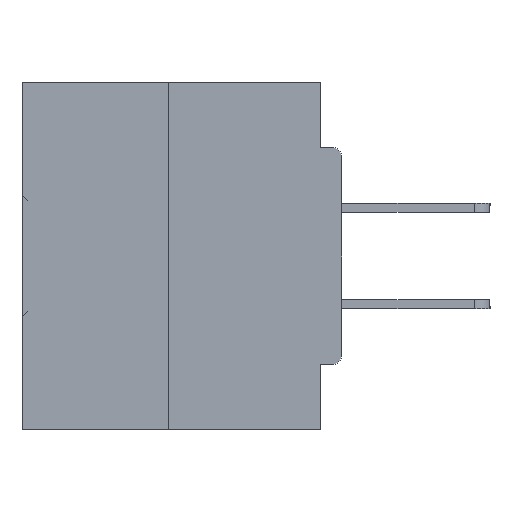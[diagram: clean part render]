
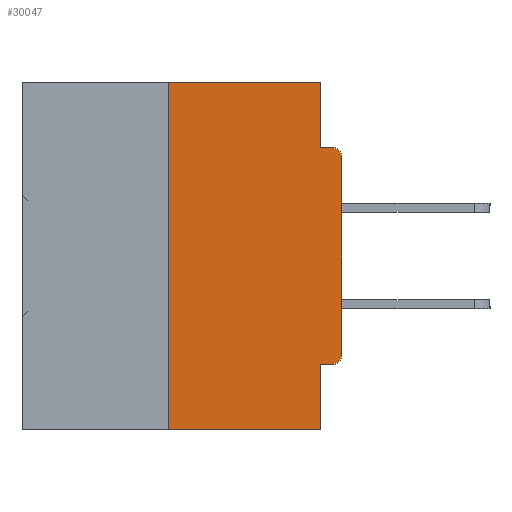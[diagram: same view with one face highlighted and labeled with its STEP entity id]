
A CAD part, left-side view. The second image highlights one B-rep face of the part: STEP entity #30047.
In plain terms, the highlighted planar face has unit normal (-1, 0, 0).
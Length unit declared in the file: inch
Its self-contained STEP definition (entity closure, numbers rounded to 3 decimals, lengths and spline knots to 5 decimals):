
#75 = ORIENTED_EDGE ( 'NONE', *, *, #35753, .F. ) ;
#793 = CARTESIAN_POINT ( 'NONE',  ( 0., 0.031, -0.0935 ) ) ;
#1240 = DIRECTION ( 'NONE',  ( 0., 0., 1. ) ) ;
#2278 = LINE ( 'NONE', #16675, #15530 ) ;
#2616 = VECTOR ( 'NONE', #43213, 39.37008 ) ;
#3412 = EDGE_CURVE ( 'NONE', #6064, #9976, #33629, .T. ) ;
#3781 = VECTOR ( 'NONE', #18982, 39.37008 ) ;
#4092 = CARTESIAN_POINT ( 'NONE',  ( 0., 0.25, 0. ) ) ;
#4139 = DIRECTION ( 'NONE',  ( 0., -1., 0. ) ) ;
#4508 = VERTEX_POINT ( 'NONE', #6081 ) ;
#4993 = CARTESIAN_POINT ( 'NONE',  ( 0., 0.25, 0. ) ) ;
#5034 = CARTESIAN_POINT ( 'NONE',  ( 0., 0., -0.3915 ) ) ;
#5086 = DIRECTION ( 'NONE',  ( 0., 1., 0. ) ) ;
#5139 = FACE_OUTER_BOUND ( 'NONE', #24367, .T. ) ;
#5368 = DIRECTION ( 'NONE',  ( 0., 0., -1. ) ) ;
#6064 = VERTEX_POINT ( 'NONE', #5034 ) ;
#6081 = CARTESIAN_POINT ( 'NONE',  ( 0., 0.25, -0.5 ) ) ;
#7770 = EDGE_CURVE ( 'NONE', #8188, #32114, #13104, .T. ) ;
#7917 = LINE ( 'NONE', #37010, #18830 ) ;
#8063 = VERTEX_POINT ( 'NONE', #11401 ) ;
#8188 = VERTEX_POINT ( 'NONE', #22750 ) ;
#8562 = ORIENTED_EDGE ( 'NONE', *, *, #7770, .F. ) ;
#8896 = CIRCLE ( 'NONE', #14152, 0.015 ) ;
#9626 = DIRECTION ( 'NONE',  ( 1., 0., 0. ) ) ;
#9976 = VERTEX_POINT ( 'NONE', #10866 ) ;
#10424 = DIRECTION ( 'NONE',  ( -1., 0., 0. ) ) ;
#10453 = CARTESIAN_POINT ( 'NONE',  ( 0., 0.015, -0.3915 ) ) ;
#10866 = CARTESIAN_POINT ( 'NONE',  ( 0., 0., -0.1085 ) ) ;
#11401 = CARTESIAN_POINT ( 'NONE',  ( 0., 0.031, -0.5 ) ) ;
#12155 = VECTOR ( 'NONE', #5086, 39.37008 ) ;
#12430 = ORIENTED_EDGE ( 'NONE', *, *, #3412, .T. ) ;
#13104 = LINE ( 'NONE', #37975, #12155 ) ;
#13108 = EDGE_CURVE ( 'NONE', #21368, #27125, #28758, .T. ) ;
#13872 = CIRCLE ( 'NONE', #43394, 0.015 ) ;
#14152 = AXIS2_PLACEMENT_3D ( 'NONE', #24622, #10424, #43067 ) ;
#14954 = EDGE_CURVE ( 'NONE', #4508, #8063, #7917, .T. ) ;
#14983 = CARTESIAN_POINT ( 'NONE',  ( 0., 0.031, 0. ) ) ;
#15158 = DIRECTION ( 'NONE',  ( 0., 0., -1. ) ) ;
#15449 = EDGE_CURVE ( 'NONE', #27125, #32962, #36286, .T. ) ;
#15530 = VECTOR ( 'NONE', #15158, 39.37008 ) ;
#15756 = CARTESIAN_POINT ( 'NONE',  ( 0., 0.46, 0. ) ) ;
#15834 = DIRECTION ( 'NONE',  ( 0., 0., 1. ) ) ;
#16675 = CARTESIAN_POINT ( 'NONE',  ( 0., 0.031, -0.5 ) ) ;
#16897 = VECTOR ( 'NONE', #15834, 39.37008 ) ;
#18085 = VERTEX_POINT ( 'NONE', #39453 ) ;
#18830 = VECTOR ( 'NONE', #4139, 39.37008 ) ;
#18982 = DIRECTION ( 'NONE',  ( 0., 0., -1. ) ) ;
#20899 = ORIENTED_EDGE ( 'NONE', *, *, #44696, .F. ) ;
#21368 = VERTEX_POINT ( 'NONE', #4092 ) ;
#21892 = CARTESIAN_POINT ( 'NONE',  ( 0., 0.46, 0. ) ) ;
#21926 = ORIENTED_EDGE ( 'NONE', *, *, #15449, .F. ) ;
#22748 = CARTESIAN_POINT ( 'NONE',  ( 0., 0., 0. ) ) ;
#22750 = CARTESIAN_POINT ( 'NONE',  ( 0., 0.015, -0.4065 ) ) ;
#23289 = CARTESIAN_POINT ( 'NONE',  ( 0., 0.031, 0. ) ) ;
#24070 = CARTESIAN_POINT ( 'NONE',  ( 0., 0., -0.0935 ) ) ;
#24367 = EDGE_LOOP ( 'NONE', ( #28938, #75, #28077, #20899, #8562, #33001, #12430, #25408, #25571, #21926 ) ) ;
#24622 = CARTESIAN_POINT ( 'NONE',  ( 0., 0.015, -0.1085 ) ) ;
#24874 = DIRECTION ( 'NONE',  ( -1., 0., 0. ) ) ;
#25199 = VECTOR ( 'NONE', #38513, 39.37008 ) ;
#25408 = ORIENTED_EDGE ( 'NONE', *, *, #38460, .T. ) ;
#25571 = ORIENTED_EDGE ( 'NONE', *, *, #40719, .F. ) ;
#27125 = VERTEX_POINT ( 'NONE', #23289 ) ;
#28077 = ORIENTED_EDGE ( 'NONE', *, *, #14954, .T. ) ;
#28758 = LINE ( 'NONE', #21892, #2616 ) ;
#28938 = ORIENTED_EDGE ( 'NONE', *, *, #13108, .F. ) ;
#29758 = CARTESIAN_POINT ( 'NONE',  ( 0., 0.031, -0.4065 ) ) ;
#30047 = ADVANCED_FACE ( 'NONE', ( #5139 ), #37556, .F. ) ;
#32114 = VERTEX_POINT ( 'NONE', #29758 ) ;
#32962 = VERTEX_POINT ( 'NONE', #793 ) ;
#33001 = ORIENTED_EDGE ( 'NONE', *, *, #41255, .T. ) ;
#33629 = LINE ( 'NONE', #22748, #37348 ) ;
#34046 = LINE ( 'NONE', #4993, #16897 ) ;
#35753 = EDGE_CURVE ( 'NONE', #4508, #21368, #34046, .T. ) ;
#36286 = LINE ( 'NONE', #14983, #3781 ) ;
#37010 = CARTESIAN_POINT ( 'NONE',  ( 0., 0.46, -0.5 ) ) ;
#37348 = VECTOR ( 'NONE', #1240, 39.37008 ) ;
#37556 = PLANE ( 'NONE',  #45946 ) ;
#37975 = CARTESIAN_POINT ( 'NONE',  ( 0., 0., -0.4065 ) ) ;
#38460 = EDGE_CURVE ( 'NONE', #9976, #18085, #8896, .T. ) ;
#38513 = DIRECTION ( 'NONE',  ( 0., -1., 0. ) ) ;
#38747 = LINE ( 'NONE', #24070, #25199 ) ;
#39316 = DIRECTION ( 'NONE',  ( 0., 0., -1. ) ) ;
#39453 = CARTESIAN_POINT ( 'NONE',  ( 0., 0.015, -0.0935 ) ) ;
#40719 = EDGE_CURVE ( 'NONE', #32962, #18085, #38747, .T. ) ;
#41255 = EDGE_CURVE ( 'NONE', #8188, #6064, #13872, .T. ) ;
#43067 = DIRECTION ( 'NONE',  ( 0., 0., -1. ) ) ;
#43213 = DIRECTION ( 'NONE',  ( 0., -1., 0. ) ) ;
#43394 = AXIS2_PLACEMENT_3D ( 'NONE', #10453, #24874, #39316 ) ;
#44696 = EDGE_CURVE ( 'NONE', #32114, #8063, #2278, .T. ) ;
#45946 = AXIS2_PLACEMENT_3D ( 'NONE', #15756, #9626, #5368 ) ;
